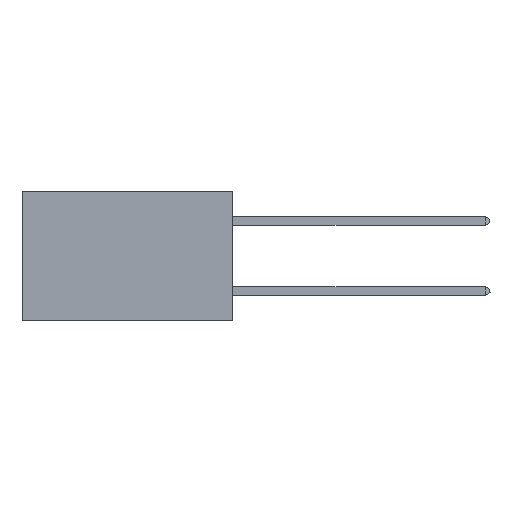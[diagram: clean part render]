
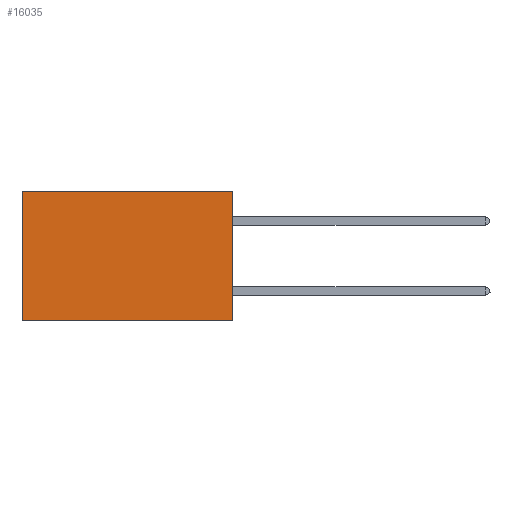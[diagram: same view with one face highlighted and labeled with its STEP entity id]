
A CAD part, left-side view. The second image highlights one B-rep face of the part: STEP entity #16035.
In plain terms, the highlighted planar face has unit normal (-1, 0, 0).
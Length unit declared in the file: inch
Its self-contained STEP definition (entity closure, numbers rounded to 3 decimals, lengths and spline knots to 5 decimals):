
#276 = DIRECTION ( 'NONE',  ( 0., 1., 0. ) ) ;
#2515 = VERTEX_POINT ( 'NONE', #21250 ) ;
#2800 = CARTESIAN_POINT ( 'NONE',  ( 0.2875, 0., 0. ) ) ;
#4258 = LINE ( 'NONE', #10890, #14005 ) ;
#4278 = LINE ( 'NONE', #7192, #15649 ) ;
#5191 = DIRECTION ( 'NONE',  ( 0., 1., 0. ) ) ;
#5369 = VERTEX_POINT ( 'NONE', #10984 ) ;
#5645 = ORIENTED_EDGE ( 'NONE', *, *, #12477, .F. ) ;
#7192 = CARTESIAN_POINT ( 'NONE',  ( 0.2875, 0.6, 0. ) ) ;
#8706 = ORIENTED_EDGE ( 'NONE', *, *, #15777, .T. ) ;
#10619 = DIRECTION ( 'NONE',  ( 1., 0., 0. ) ) ;
#10828 = AXIS2_PLACEMENT_3D ( 'NONE', #17092, #10619, #19071 ) ;
#10890 = CARTESIAN_POINT ( 'NONE',  ( 0.2875, 0., -0.37 ) ) ;
#10984 = CARTESIAN_POINT ( 'NONE',  ( 0.2875, 0.6, -0.37 ) ) ;
#12477 = EDGE_CURVE ( 'NONE', #24770, #20848, #18857, .T. ) ;
#12613 = EDGE_CURVE ( 'NONE', #20848, #5369, #4258, .T. ) ;
#13195 = DIRECTION ( 'NONE',  ( 0., 0., -1. ) ) ;
#14005 = VECTOR ( 'NONE', #276, 39.37008 ) ;
#14356 = CARTESIAN_POINT ( 'NONE',  ( 0.2875, 0., 0. ) ) ;
#15649 = VECTOR ( 'NONE', #13195, 39.37008 ) ;
#15777 = EDGE_CURVE ( 'NONE', #24770, #2515, #17101, .T. ) ;
#16035 = ADVANCED_FACE ( 'NONE', ( #19654 ), #23133, .F. ) ;
#16742 = CARTESIAN_POINT ( 'NONE',  ( 0.2875, 0., -0.37 ) ) ;
#17092 = CARTESIAN_POINT ( 'NONE',  ( 0.2875, 0., 0. ) ) ;
#17101 = LINE ( 'NONE', #26210, #26483 ) ;
#18622 = EDGE_CURVE ( 'NONE', #2515, #5369, #4278, .T. ) ;
#18857 = LINE ( 'NONE', #14356, #25988 ) ;
#19071 = DIRECTION ( 'NONE',  ( 0., 0., -1. ) ) ;
#19654 = FACE_OUTER_BOUND ( 'NONE', #26543, .T. ) ;
#20848 = VERTEX_POINT ( 'NONE', #16742 ) ;
#21250 = CARTESIAN_POINT ( 'NONE',  ( 0.2875, 0.6, 0. ) ) ;
#22603 = DIRECTION ( 'NONE',  ( 0., 0., -1. ) ) ;
#23133 = PLANE ( 'NONE',  #10828 ) ;
#24309 = ORIENTED_EDGE ( 'NONE', *, *, #12613, .F. ) ;
#24770 = VERTEX_POINT ( 'NONE', #2800 ) ;
#25988 = VECTOR ( 'NONE', #22603, 39.37008 ) ;
#26210 = CARTESIAN_POINT ( 'NONE',  ( 0.2875, 0., 0. ) ) ;
#26483 = VECTOR ( 'NONE', #5191, 39.37008 ) ;
#26543 = EDGE_LOOP ( 'NONE', ( #26570, #24309, #5645, #8706 ) ) ;
#26570 = ORIENTED_EDGE ( 'NONE', *, *, #18622, .T. ) ;
